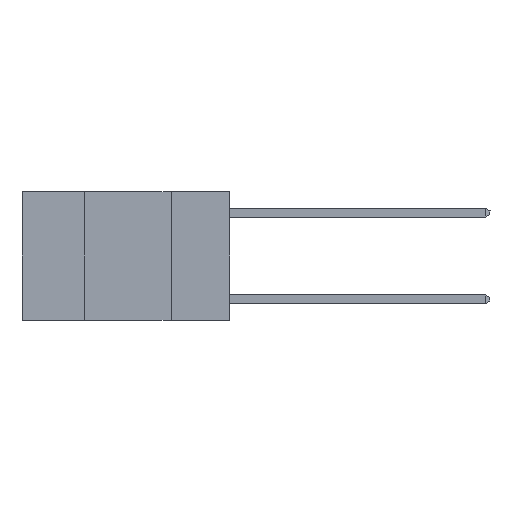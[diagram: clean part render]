
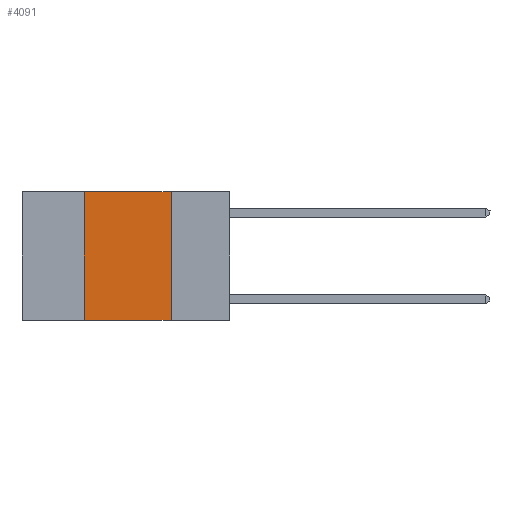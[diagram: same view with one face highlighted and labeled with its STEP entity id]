
A CAD part, left-side view. The second image highlights one B-rep face of the part: STEP entity #4091.
In plain terms, the highlighted planar face has unit normal (-1, 0, 0).
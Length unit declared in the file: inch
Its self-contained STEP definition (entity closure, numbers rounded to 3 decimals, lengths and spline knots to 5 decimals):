
#128 = VERTEX_POINT ( 'NONE', #7501 ) ;
#288 = VERTEX_POINT ( 'NONE', #2940 ) ;
#490 = DIRECTION ( 'NONE',  ( 0., 0., 1. ) ) ;
#580 = CARTESIAN_POINT ( 'NONE',  ( 0., 0.17, 0. ) ) ;
#1154 = EDGE_LOOP ( 'NONE', ( #1923, #2082, #2225, #2311 ) ) ;
#1459 = CARTESIAN_POINT ( 'NONE',  ( 0., 0.6, 0. ) ) ;
#1586 = DIRECTION ( 'NONE',  ( 0., -1., 0. ) ) ;
#1772 = EDGE_CURVE ( 'NONE', #288, #3458, #4003, .T. ) ;
#1923 = ORIENTED_EDGE ( 'NONE', *, *, #8014, .F. ) ;
#2082 = ORIENTED_EDGE ( 'NONE', *, *, #10074, .F. ) ;
#2093 = AXIS2_PLACEMENT_3D ( 'NONE', #1459, #10019, #4941 ) ;
#2225 = ORIENTED_EDGE ( 'NONE', *, *, #10434, .F. ) ;
#2311 = ORIENTED_EDGE ( 'NONE', *, *, #1772, .T. ) ;
#2940 = CARTESIAN_POINT ( 'NONE',  ( 0., 0.42, -0.37 ) ) ;
#3147 = PLANE ( 'NONE',  #2093 ) ;
#3150 = DIRECTION ( 'NONE',  ( 0., 0., -1. ) ) ;
#3458 = VERTEX_POINT ( 'NONE', #5976 ) ;
#4003 = LINE ( 'NONE', #10994, #6041 ) ;
#4091 = ADVANCED_FACE ( 'NONE', ( #4923 ), #3147, .F. ) ;
#4099 = VERTEX_POINT ( 'NONE', #580 ) ;
#4180 = DIRECTION ( 'NONE',  ( 0., -1., 0. ) ) ;
#4335 = VECTOR ( 'NONE', #490, 39.37008 ) ;
#4606 = LINE ( 'NONE', #8292, #4335 ) ;
#4923 = FACE_OUTER_BOUND ( 'NONE', #1154, .T. ) ;
#4941 = DIRECTION ( 'NONE',  ( 0., 0., -1. ) ) ;
#5617 = LINE ( 'NONE', #9114, #9856 ) ;
#5976 = CARTESIAN_POINT ( 'NONE',  ( 0., 0.17, -0.37 ) ) ;
#6041 = VECTOR ( 'NONE', #1586, 39.37008 ) ;
#6365 = VECTOR ( 'NONE', #4180, 39.37008 ) ;
#6629 = LINE ( 'NONE', #6750, #6365 ) ;
#6750 = CARTESIAN_POINT ( 'NONE',  ( 0., 0.6, 0. ) ) ;
#7501 = CARTESIAN_POINT ( 'NONE',  ( 0., 0.42, 0. ) ) ;
#8014 = EDGE_CURVE ( 'NONE', #4099, #3458, #5617, .T. ) ;
#8292 = CARTESIAN_POINT ( 'NONE',  ( 0., 0.42, 0. ) ) ;
#9114 = CARTESIAN_POINT ( 'NONE',  ( 0., 0.17, 0. ) ) ;
#9856 = VECTOR ( 'NONE', #3150, 39.37008 ) ;
#10019 = DIRECTION ( 'NONE',  ( 1., 0., 0. ) ) ;
#10074 = EDGE_CURVE ( 'NONE', #128, #4099, #6629, .T. ) ;
#10434 = EDGE_CURVE ( 'NONE', #288, #128, #4606, .T. ) ;
#10994 = CARTESIAN_POINT ( 'NONE',  ( 0., 0.6, -0.37 ) ) ;
